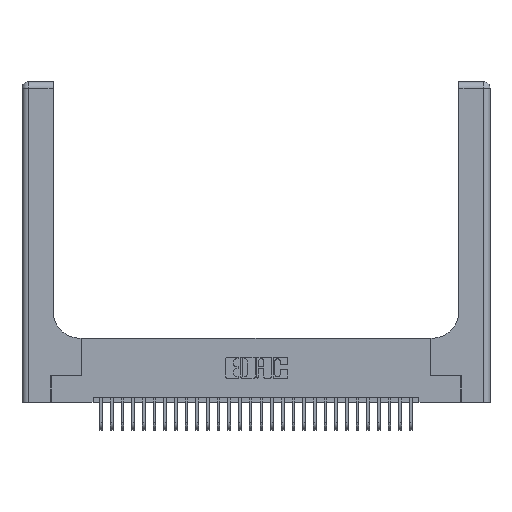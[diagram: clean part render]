
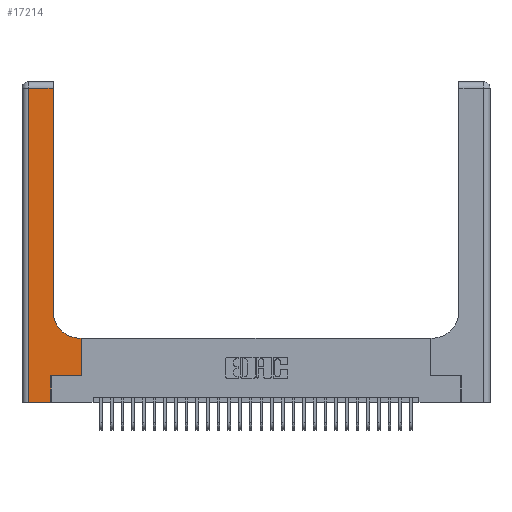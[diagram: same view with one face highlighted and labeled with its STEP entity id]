
A CAD part, top view. The second image highlights one B-rep face of the part: STEP entity #17214.
In plain terms, the highlighted planar face has unit normal (0, 0, 1).
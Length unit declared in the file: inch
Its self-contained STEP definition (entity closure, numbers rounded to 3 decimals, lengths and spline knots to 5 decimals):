
#287 = CARTESIAN_POINT ( 'NONE',  ( 0.269, 0., 0.37 ) ) ;
#974 = VECTOR ( 'NONE', #6545, 39.37008 ) ;
#1322 = ORIENTED_EDGE ( 'NONE', *, *, #13837, .T. ) ;
#1985 = CARTESIAN_POINT ( 'NONE',  ( 0.2915, 0.85, 0.37 ) ) ;
#2377 = VECTOR ( 'NONE', #11797, 39.37008 ) ;
#2612 = LINE ( 'NONE', #27492, #14073 ) ;
#3524 = CIRCLE ( 'NONE', #11400, 0.25 ) ;
#3537 = EDGE_CURVE ( 'NONE', #27445, #9761, #3524, .T. ) ;
#3926 = CARTESIAN_POINT ( 'NONE',  ( 0.269, 0.25, 0.37 ) ) ;
#4052 = EDGE_CURVE ( 'NONE', #8386, #6731, #20191, .T. ) ;
#4096 = LINE ( 'NONE', #10652, #22208 ) ;
#4130 = CARTESIAN_POINT ( 'NONE',  ( 0.269, 0., 0.37 ) ) ;
#4348 = DIRECTION ( 'NONE',  ( 0., 0., -1. ) ) ;
#5004 = DIRECTION ( 'NONE',  ( 0., 0., -1. ) ) ;
#5452 = EDGE_CURVE ( 'NONE', #15577, #16727, #13424, .T. ) ;
#5497 = CARTESIAN_POINT ( 'NONE',  ( 0.269, 0.25, 0.37 ) ) ;
#6545 = DIRECTION ( 'NONE',  ( 0., 1., 0. ) ) ;
#6731 = VERTEX_POINT ( 'NONE', #17238 ) ;
#6988 = FACE_OUTER_BOUND ( 'NONE', #10190, .T. ) ;
#7157 = LINE ( 'NONE', #4130, #974 ) ;
#7578 = ORIENTED_EDGE ( 'NONE', *, *, #17377, .T. ) ;
#8071 = VERTEX_POINT ( 'NONE', #11082 ) ;
#8107 = VECTOR ( 'NONE', #9381, 39.37008 ) ;
#8386 = VERTEX_POINT ( 'NONE', #5497 ) ;
#9238 = ORIENTED_EDGE ( 'NONE', *, *, #22906, .T. ) ;
#9381 = DIRECTION ( 'NONE',  ( 1., 0., 0. ) ) ;
#9761 = VERTEX_POINT ( 'NONE', #1985 ) ;
#10190 = EDGE_LOOP ( 'NONE', ( #9238, #7578, #21490, #19292, #1322, #14581, #13528, #12295, #17727 ) ) ;
#10452 = CARTESIAN_POINT ( 'NONE',  ( 0.06, 2.94, 0.37 ) ) ;
#10652 = CARTESIAN_POINT ( 'NONE',  ( 0.5585, 0.25, 0.37 ) ) ;
#11082 = CARTESIAN_POINT ( 'NONE',  ( 0.2915, 2.94, 0.37 ) ) ;
#11400 = AXIS2_PLACEMENT_3D ( 'NONE', #18549, #5004, #20848 ) ;
#11527 = DIRECTION ( 'NONE',  ( 0., 1., 0. ) ) ;
#11783 = VERTEX_POINT ( 'NONE', #10452 ) ;
#11797 = DIRECTION ( 'NONE',  ( 0., -1., 0. ) ) ;
#12295 = ORIENTED_EDGE ( 'NONE', *, *, #21626, .T. ) ;
#13081 = DIRECTION ( 'NONE',  ( -1., 0., 0. ) ) ;
#13424 = LINE ( 'NONE', #16089, #8107 ) ;
#13528 = ORIENTED_EDGE ( 'NONE', *, *, #19273, .T. ) ;
#13837 = EDGE_CURVE ( 'NONE', #16727, #8386, #7157, .T. ) ;
#14073 = VECTOR ( 'NONE', #16271, 39.37008 ) ;
#14581 = ORIENTED_EDGE ( 'NONE', *, *, #4052, .T. ) ;
#14654 = VECTOR ( 'NONE', #13081, 39.37008 ) ;
#15577 = VERTEX_POINT ( 'NONE', #18108 ) ;
#16089 = CARTESIAN_POINT ( 'NONE',  ( 0., 0., 0.37 ) ) ;
#16271 = DIRECTION ( 'NONE',  ( -1., 0., 0. ) ) ;
#16727 = VERTEX_POINT ( 'NONE', #287 ) ;
#17214 = ADVANCED_FACE ( 'NONE', ( #6988 ), #20098, .F. ) ;
#17238 = CARTESIAN_POINT ( 'NONE',  ( 0.5585, 0.25, 0.37 ) ) ;
#17377 = EDGE_CURVE ( 'NONE', #8071, #11783, #2612, .T. ) ;
#17727 = ORIENTED_EDGE ( 'NONE', *, *, #3537, .T. ) ;
#17902 = VERTEX_POINT ( 'NONE', #27165 ) ;
#17917 = CARTESIAN_POINT ( 'NONE',  ( 0., 3., 0.37 ) ) ;
#18036 = AXIS2_PLACEMENT_3D ( 'NONE', #17917, #4348, #20198 ) ;
#18108 = CARTESIAN_POINT ( 'NONE',  ( 0.06, 0., 0.37 ) ) ;
#18473 = CARTESIAN_POINT ( 'NONE',  ( 0.06, 3., 0.37 ) ) ;
#18549 = CARTESIAN_POINT ( 'NONE',  ( 0.5415, 0.85, 0.37 ) ) ;
#19273 = EDGE_CURVE ( 'NONE', #6731, #17902, #4096, .T. ) ;
#19292 = ORIENTED_EDGE ( 'NONE', *, *, #5452, .T. ) ;
#19489 = VECTOR ( 'NONE', #26594, 39.37008 ) ;
#19910 = LINE ( 'NONE', #28829, #14654 ) ;
#20098 = PLANE ( 'NONE',  #18036 ) ;
#20191 = LINE ( 'NONE', #3926, #19489 ) ;
#20198 = DIRECTION ( 'NONE',  ( -1., 0., 0. ) ) ;
#20498 = CARTESIAN_POINT ( 'NONE',  ( 0.2915, 3., 0.37 ) ) ;
#20848 = DIRECTION ( 'NONE',  ( 1., 0., 0. ) ) ;
#21490 = ORIENTED_EDGE ( 'NONE', *, *, #26665, .T. ) ;
#21626 = EDGE_CURVE ( 'NONE', #17902, #27445, #19910, .T. ) ;
#21676 = VECTOR ( 'NONE', #11527, 39.37008 ) ;
#21980 = LINE ( 'NONE', #18473, #2377 ) ;
#22208 = VECTOR ( 'NONE', #24141, 39.37008 ) ;
#22906 = EDGE_CURVE ( 'NONE', #9761, #8071, #28348, .T. ) ;
#23396 = CARTESIAN_POINT ( 'NONE',  ( 0.5415, 0.6, 0.37 ) ) ;
#24141 = DIRECTION ( 'NONE',  ( 0., 1., 0. ) ) ;
#26594 = DIRECTION ( 'NONE',  ( 1., 0., 0. ) ) ;
#26665 = EDGE_CURVE ( 'NONE', #11783, #15577, #21980, .T. ) ;
#27165 = CARTESIAN_POINT ( 'NONE',  ( 0.5585, 0.6, 0.37 ) ) ;
#27445 = VERTEX_POINT ( 'NONE', #23396 ) ;
#27492 = CARTESIAN_POINT ( 'NONE',  ( 0., 2.94, 0.37 ) ) ;
#28348 = LINE ( 'NONE', #20498, #21676 ) ;
#28829 = CARTESIAN_POINT ( 'NONE',  ( 0.2915, 0.6, 0.37 ) ) ;
